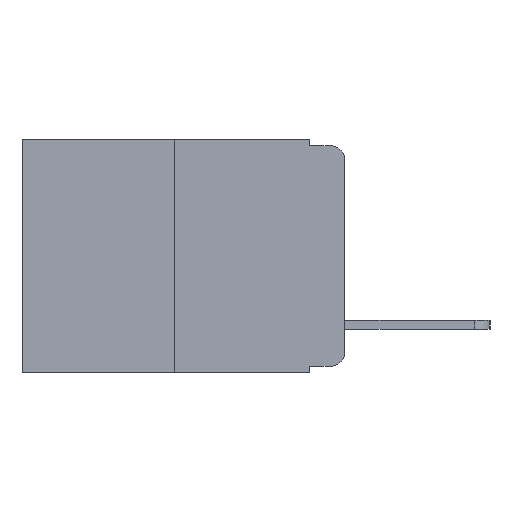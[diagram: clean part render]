
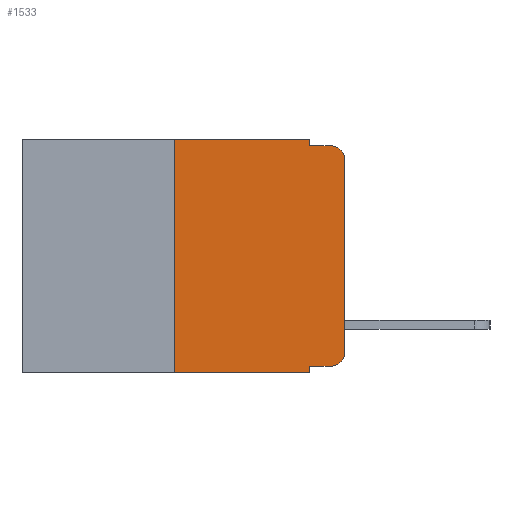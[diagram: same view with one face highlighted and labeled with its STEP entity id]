
A CAD part, left-side view. The second image highlights one B-rep face of the part: STEP entity #1533.
In plain terms, the highlighted planar face has unit normal (-1, 0, 0).
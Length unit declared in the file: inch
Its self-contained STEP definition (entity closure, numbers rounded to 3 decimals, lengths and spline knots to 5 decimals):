
#262 = ORIENTED_EDGE ( 'NONE', *, *, #6871, .T. ) ;
#516 = VERTEX_POINT ( 'NONE', #9815 ) ;
#562 = LINE ( 'NONE', #9631, #12123 ) ;
#717 = CARTESIAN_POINT ( 'NONE',  ( 0., 0.25, 0. ) ) ;
#729 = VERTEX_POINT ( 'NONE', #717 ) ;
#851 = LINE ( 'NONE', #2122, #6677 ) ;
#1036 = ORIENTED_EDGE ( 'NONE', *, *, #5299, .F. ) ;
#1440 = FACE_OUTER_BOUND ( 'NONE', #9434, .T. ) ;
#1533 = ADVANCED_FACE ( 'NONE', ( #1440 ), #6052, .F. ) ;
#1609 = VERTEX_POINT ( 'NONE', #4185 ) ;
#1679 = DIRECTION ( 'NONE',  ( 0., 0., -1. ) ) ;
#1890 = EDGE_CURVE ( 'NONE', #1609, #3873, #6867, .T. ) ;
#1931 = CARTESIAN_POINT ( 'NONE',  ( 0., 0.051, 0. ) ) ;
#1943 = VECTOR ( 'NONE', #9553, 39.37008 ) ;
#1983 = LINE ( 'NONE', #2879, #7314 ) ;
#2122 = CARTESIAN_POINT ( 'NONE',  ( 0., 0.051, 0. ) ) ;
#2219 = DIRECTION ( 'NONE',  ( 0., 0., -1. ) ) ;
#2236 = AXIS2_PLACEMENT_3D ( 'NONE', #12053, #12023, #12019 ) ;
#2263 = DIRECTION ( 'NONE',  ( -1., 0., 0. ) ) ;
#2264 = CARTESIAN_POINT ( 'NONE',  ( 0., 0.02, -0.313 ) ) ;
#2563 = VECTOR ( 'NONE', #11150, 39.37008 ) ;
#2756 = CARTESIAN_POINT ( 'NONE',  ( 0., 0.02, -0.333 ) ) ;
#2879 = CARTESIAN_POINT ( 'NONE',  ( 0., 0.051, 0. ) ) ;
#3087 = ORIENTED_EDGE ( 'NONE', *, *, #3670, .F. ) ;
#3100 = DIRECTION ( 'NONE',  ( 0., 0., -1. ) ) ;
#3157 = VERTEX_POINT ( 'NONE', #2756 ) ;
#3366 = ORIENTED_EDGE ( 'NONE', *, *, #4901, .F. ) ;
#3386 = DIRECTION ( 'NONE',  ( 0., 0., 1. ) ) ;
#3670 = EDGE_CURVE ( 'NONE', #729, #10329, #562, .T. ) ;
#3859 = CARTESIAN_POINT ( 'NONE',  ( 0., 0.25, 0. ) ) ;
#3873 = VERTEX_POINT ( 'NONE', #10587 ) ;
#3884 = VERTEX_POINT ( 'NONE', #9415 ) ;
#4185 = CARTESIAN_POINT ( 'NONE',  ( 0., 0.25, -0.343 ) ) ;
#4901 = EDGE_CURVE ( 'NONE', #10471, #3873, #1983, .T. ) ;
#4943 = EDGE_CURVE ( 'NONE', #10329, #3884, #851, .T. ) ;
#5244 = ORIENTED_EDGE ( 'NONE', *, *, #6688, .T. ) ;
#5286 = VECTOR ( 'NONE', #3386, 39.37008 ) ;
#5299 = EDGE_CURVE ( 'NONE', #1609, #729, #5632, .T. ) ;
#5509 = DIRECTION ( 'NONE',  ( 0., -1., 0. ) ) ;
#5526 = AXIS2_PLACEMENT_3D ( 'NONE', #7476, #7448, #7407 ) ;
#5632 = LINE ( 'NONE', #3859, #5286 ) ;
#5724 = EDGE_CURVE ( 'NONE', #10471, #3157, #8658, .T. ) ;
#6052 = PLANE ( 'NONE',  #5526 ) ;
#6092 = CARTESIAN_POINT ( 'NONE',  ( 0., 0., -0.03 ) ) ;
#6408 = EDGE_CURVE ( 'NONE', #3157, #6636, #11724, .T. ) ;
#6636 = VERTEX_POINT ( 'NONE', #10785 ) ;
#6677 = VECTOR ( 'NONE', #1679, 39.37008 ) ;
#6688 = EDGE_CURVE ( 'NONE', #6636, #7444, #11945, .T. ) ;
#6867 = LINE ( 'NONE', #9923, #11225 ) ;
#6871 = EDGE_CURVE ( 'NONE', #7444, #516, #10037, .T. ) ;
#6991 = EDGE_CURVE ( 'NONE', #3884, #516, #8361, .T. ) ;
#7314 = VECTOR ( 'NONE', #3100, 39.37008 ) ;
#7407 = DIRECTION ( 'NONE',  ( 0., 0., -1. ) ) ;
#7444 = VERTEX_POINT ( 'NONE', #6092 ) ;
#7448 = DIRECTION ( 'NONE',  ( 1., 0., 0. ) ) ;
#7476 = CARTESIAN_POINT ( 'NONE',  ( 0., 0.473, 0. ) ) ;
#7630 = ORIENTED_EDGE ( 'NONE', *, *, #4943, .F. ) ;
#8361 = LINE ( 'NONE', #11171, #2563 ) ;
#8608 = CARTESIAN_POINT ( 'NONE',  ( 0., 0., 0. ) ) ;
#8658 = LINE ( 'NONE', #9516, #1943 ) ;
#8678 = DIRECTION ( 'NONE',  ( 0., 0., 1. ) ) ;
#8802 = ORIENTED_EDGE ( 'NONE', *, *, #6408, .T. ) ;
#9320 = CARTESIAN_POINT ( 'NONE',  ( 0., 0.051, -0.333 ) ) ;
#9415 = CARTESIAN_POINT ( 'NONE',  ( 0., 0.051, -0.01 ) ) ;
#9434 = EDGE_LOOP ( 'NONE', ( #5244, #262, #9650, #7630, #3087, #1036, #10026, #3366, #9942, #8802 ) ) ;
#9516 = CARTESIAN_POINT ( 'NONE',  ( 0., 0.051, -0.333 ) ) ;
#9553 = DIRECTION ( 'NONE',  ( 0., -1., 0. ) ) ;
#9631 = CARTESIAN_POINT ( 'NONE',  ( 0., 0.473, 0. ) ) ;
#9650 = ORIENTED_EDGE ( 'NONE', *, *, #6991, .F. ) ;
#9815 = CARTESIAN_POINT ( 'NONE',  ( 0., 0.02, -0.01 ) ) ;
#9923 = CARTESIAN_POINT ( 'NONE',  ( 0., 0.473, -0.343 ) ) ;
#9942 = ORIENTED_EDGE ( 'NONE', *, *, #5724, .T. ) ;
#10026 = ORIENTED_EDGE ( 'NONE', *, *, #1890, .T. ) ;
#10037 = CIRCLE ( 'NONE', #2236, 0.02 ) ;
#10329 = VERTEX_POINT ( 'NONE', #1931 ) ;
#10471 = VERTEX_POINT ( 'NONE', #9320 ) ;
#10525 = AXIS2_PLACEMENT_3D ( 'NONE', #2264, #2263, #2219 ) ;
#10587 = CARTESIAN_POINT ( 'NONE',  ( 0., 0.051, -0.343 ) ) ;
#10785 = CARTESIAN_POINT ( 'NONE',  ( 0., 0., -0.313 ) ) ;
#10928 = DIRECTION ( 'NONE',  ( 0., -1., 0. ) ) ;
#11150 = DIRECTION ( 'NONE',  ( 0., -1., 0. ) ) ;
#11171 = CARTESIAN_POINT ( 'NONE',  ( 0., 0.051, -0.01 ) ) ;
#11225 = VECTOR ( 'NONE', #10928, 39.37008 ) ;
#11714 = VECTOR ( 'NONE', #8678, 39.37008 ) ;
#11724 = CIRCLE ( 'NONE', #10525, 0.02 ) ;
#11945 = LINE ( 'NONE', #8608, #11714 ) ;
#12019 = DIRECTION ( 'NONE',  ( 0., 0., -1. ) ) ;
#12023 = DIRECTION ( 'NONE',  ( -1., 0., 0. ) ) ;
#12053 = CARTESIAN_POINT ( 'NONE',  ( 0., 0.02, -0.03 ) ) ;
#12123 = VECTOR ( 'NONE', #5509, 39.37008 ) ;
